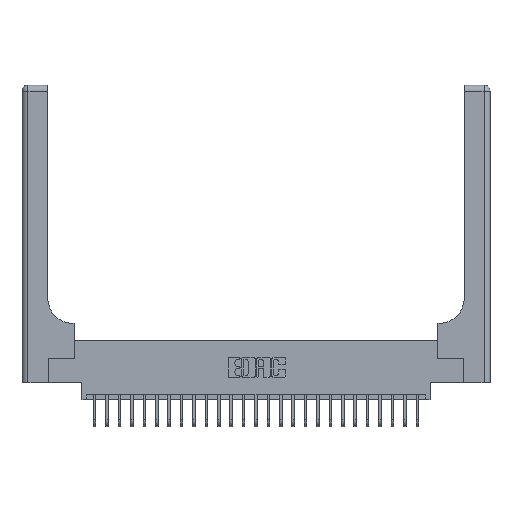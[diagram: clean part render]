
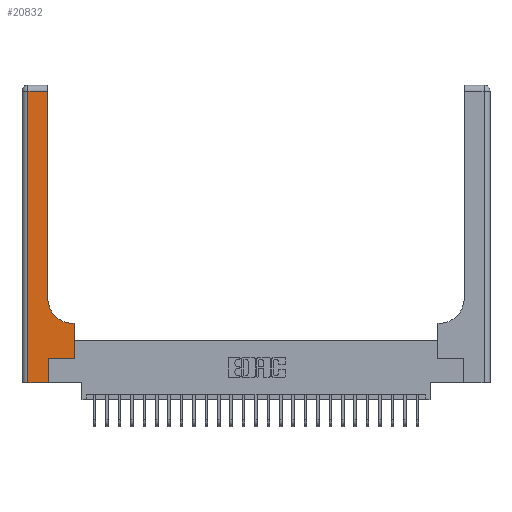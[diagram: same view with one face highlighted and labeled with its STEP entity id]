
A CAD part, top view. The second image highlights one B-rep face of the part: STEP entity #20832.
In plain terms, the highlighted planar face has unit normal (0, 0, 1).
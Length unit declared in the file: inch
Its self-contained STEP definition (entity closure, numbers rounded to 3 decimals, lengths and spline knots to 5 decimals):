
#403 = EDGE_CURVE ( 'NONE', #19942, #4212, #10443, .T. ) ;
#462 = ORIENTED_EDGE ( 'NONE', *, *, #26298, .T. ) ;
#1135 = CARTESIAN_POINT ( 'NONE',  ( 0.26, 3., 0.37 ) ) ;
#1517 = ORIENTED_EDGE ( 'NONE', *, *, #403, .T. ) ;
#1752 = EDGE_CURVE ( 'NONE', #5525, #3000, #18524, .T. ) ;
#1770 = VECTOR ( 'NONE', #21150, 39.37008 ) ;
#2053 = EDGE_CURVE ( 'NONE', #22274, #19942, #17687, .T. ) ;
#2585 = CARTESIAN_POINT ( 'NONE',  ( 0.26, 2.94, 0.37 ) ) ;
#2615 = CARTESIAN_POINT ( 'NONE',  ( 0.528, 0.25, 0.37 ) ) ;
#3000 = VERTEX_POINT ( 'NONE', #22375 ) ;
#3298 = CARTESIAN_POINT ( 'NONE',  ( 0.265, 0.25, 0.37 ) ) ;
#3824 = DIRECTION ( 'NONE',  ( 0., 0., -1. ) ) ;
#3861 = VECTOR ( 'NONE', #15619, 39.37008 ) ;
#3901 = DIRECTION ( 'NONE',  ( -1., 0., 0. ) ) ;
#4212 = VERTEX_POINT ( 'NONE', #13234 ) ;
#4598 = LINE ( 'NONE', #6543, #22421 ) ;
#5414 = DIRECTION ( 'NONE',  ( 0., 1., 0. ) ) ;
#5524 = EDGE_CURVE ( 'NONE', #6519, #24838, #18187, .T. ) ;
#5525 = VERTEX_POINT ( 'NONE', #14054 ) ;
#6268 = AXIS2_PLACEMENT_3D ( 'NONE', #26949, #3824, #12264 ) ;
#6519 = VERTEX_POINT ( 'NONE', #3298 ) ;
#6543 = CARTESIAN_POINT ( 'NONE',  ( 0., 2.94, 0.37 ) ) ;
#6695 = FACE_OUTER_BOUND ( 'NONE', #8647, .T. ) ;
#6864 = VERTEX_POINT ( 'NONE', #2585 ) ;
#6897 = CARTESIAN_POINT ( 'NONE',  ( 0.06, 0., 0.37 ) ) ;
#7122 = CARTESIAN_POINT ( 'NONE',  ( 0.265, 0., 0.37 ) ) ;
#7774 = VERTEX_POINT ( 'NONE', #10373 ) ;
#8245 = ORIENTED_EDGE ( 'NONE', *, *, #1752, .T. ) ;
#8647 = EDGE_LOOP ( 'NONE', ( #24402, #462, #14092, #1517, #13835, #19675, #22532, #8245, #19803 ) ) ;
#9672 = DIRECTION ( 'NONE',  ( 1., 0., 0. ) ) ;
#9704 = LINE ( 'NONE', #1135, #22155 ) ;
#10373 = CARTESIAN_POINT ( 'NONE',  ( 0.26, 0.85, 0.37 ) ) ;
#10443 = LINE ( 'NONE', #16757, #1770 ) ;
#12141 = CARTESIAN_POINT ( 'NONE',  ( 0.265, 0.25, 0.37 ) ) ;
#12264 = DIRECTION ( 'NONE',  ( 1., 0., 0. ) ) ;
#12915 = CARTESIAN_POINT ( 'NONE',  ( 0., 3., 0.37 ) ) ;
#13234 = CARTESIAN_POINT ( 'NONE',  ( 0.265, 0., 0.37 ) ) ;
#13835 = ORIENTED_EDGE ( 'NONE', *, *, #23404, .T. ) ;
#13952 = AXIS2_PLACEMENT_3D ( 'NONE', #12915, #21288, #25811 ) ;
#14054 = CARTESIAN_POINT ( 'NONE',  ( 0.528, 0.6, 0.37 ) ) ;
#14092 = ORIENTED_EDGE ( 'NONE', *, *, #2053, .T. ) ;
#14322 = VECTOR ( 'NONE', #3901, 39.37008 ) ;
#15619 = DIRECTION ( 'NONE',  ( 0., -1., 0. ) ) ;
#16757 = CARTESIAN_POINT ( 'NONE',  ( 0., 0., 0.37 ) ) ;
#17014 = EDGE_CURVE ( 'NONE', #3000, #7774, #18173, .T. ) ;
#17090 = DIRECTION ( 'NONE',  ( 0., 1., 0. ) ) ;
#17687 = LINE ( 'NONE', #19462, #3861 ) ;
#18173 = CIRCLE ( 'NONE', #6268, 0.25 ) ;
#18187 = LINE ( 'NONE', #12141, #18368 ) ;
#18368 = VECTOR ( 'NONE', #9672, 39.37008 ) ;
#18524 = LINE ( 'NONE', #26896, #14322 ) ;
#18613 = EDGE_CURVE ( 'NONE', #24838, #5525, #21215, .T. ) ;
#19462 = CARTESIAN_POINT ( 'NONE',  ( 0.06, 3., 0.37 ) ) ;
#19675 = ORIENTED_EDGE ( 'NONE', *, *, #5524, .T. ) ;
#19688 = EDGE_CURVE ( 'NONE', #7774, #6864, #9704, .T. ) ;
#19803 = ORIENTED_EDGE ( 'NONE', *, *, #17014, .T. ) ;
#19942 = VERTEX_POINT ( 'NONE', #6897 ) ;
#20357 = VECTOR ( 'NONE', #17090, 39.37008 ) ;
#20832 = ADVANCED_FACE ( 'NONE', ( #6695 ), #26099, .F. ) ;
#21150 = DIRECTION ( 'NONE',  ( 1., 0., 0. ) ) ;
#21215 = LINE ( 'NONE', #2615, #20357 ) ;
#21233 = CARTESIAN_POINT ( 'NONE',  ( 0.528, 0.25, 0.37 ) ) ;
#21260 = CARTESIAN_POINT ( 'NONE',  ( 0.06, 2.94, 0.37 ) ) ;
#21288 = DIRECTION ( 'NONE',  ( 0., 0., -1. ) ) ;
#22155 = VECTOR ( 'NONE', #5414, 39.37008 ) ;
#22274 = VERTEX_POINT ( 'NONE', #21260 ) ;
#22375 = CARTESIAN_POINT ( 'NONE',  ( 0.51, 0.6, 0.37 ) ) ;
#22421 = VECTOR ( 'NONE', #25252, 39.37008 ) ;
#22532 = ORIENTED_EDGE ( 'NONE', *, *, #18613, .T. ) ;
#22806 = VECTOR ( 'NONE', #25307, 39.37008 ) ;
#23404 = EDGE_CURVE ( 'NONE', #4212, #6519, #25971, .T. ) ;
#24402 = ORIENTED_EDGE ( 'NONE', *, *, #19688, .T. ) ;
#24838 = VERTEX_POINT ( 'NONE', #21233 ) ;
#25252 = DIRECTION ( 'NONE',  ( -1., 0., 0. ) ) ;
#25307 = DIRECTION ( 'NONE',  ( 0., 1., 0. ) ) ;
#25811 = DIRECTION ( 'NONE',  ( -1., 0., 0. ) ) ;
#25971 = LINE ( 'NONE', #7122, #22806 ) ;
#26099 = PLANE ( 'NONE',  #13952 ) ;
#26298 = EDGE_CURVE ( 'NONE', #6864, #22274, #4598, .T. ) ;
#26896 = CARTESIAN_POINT ( 'NONE',  ( 0.26, 0.6, 0.37 ) ) ;
#26949 = CARTESIAN_POINT ( 'NONE',  ( 0.51, 0.85, 0.37 ) ) ;
